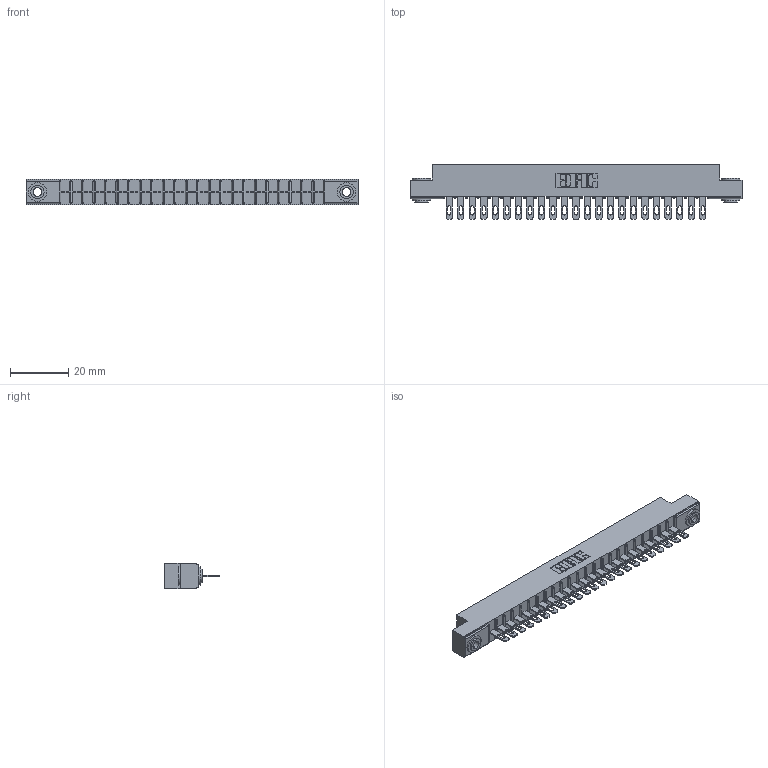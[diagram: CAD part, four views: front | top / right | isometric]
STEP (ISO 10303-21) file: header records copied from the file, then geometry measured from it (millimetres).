
FILE_DESCRIPTION (( 'STEP AP203' ), '1' );
FILE_NAME ('316-023-500-103.STEP', '2018-07-31T02:00:05', ( '' ), ( '' ), 'SwSTEP 2.0', 'SolidWorks 2016', '' );
FILE_SCHEMA (( 'CONFIG_CONTROL_DESIGN' ));
Length unit declared in the file: inch
Products named in the file (4): 345-250-002_345-250-002-102; 316-023-500-103; 306 Part_.156 Dia; 306-290-001_100
Assembly tree (26 placements, depth 2):
  316-023-500-103
    306 Part_.156 Dia
    306-290-001_100  x23
    345-250-002_345-250-002-102  x2
Bounding box: 114.15 x 18.87 x 8.71 mm (x, y, z)
Volume: 7890.5 mm3; surface area: 12306.9 mm2
Topology: 26 solids, 26 shells, 1916 faces, 5373 edges, 3454 vertices
Faces by surface type: plane 1242, cylinder 574, sphere 92, cone 8
Entity records: 25139 total; most frequent: CARTESIAN_POINT 4197, DIRECTION 4155, ORIENTED_EDGE 4150, EDGE_CURVE 2075, LINE 1603, VECTOR 1603, VERTEX_POINT 1318, AXIS2_PLACEMENT_3D 1276
